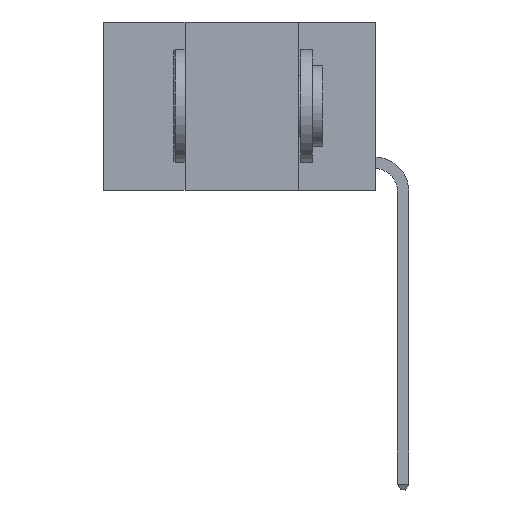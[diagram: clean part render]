
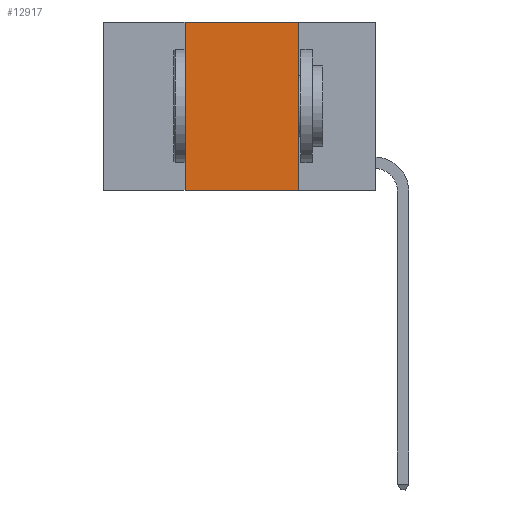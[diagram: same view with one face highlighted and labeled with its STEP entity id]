
A CAD part, left-side view. The second image highlights one B-rep face of the part: STEP entity #12917.
In plain terms, the highlighted planar face has unit normal (-1, 0, 0).
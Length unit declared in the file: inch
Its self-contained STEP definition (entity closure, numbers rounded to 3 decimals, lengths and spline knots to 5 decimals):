
#216 = VERTEX_POINT ( 'NONE', #19023 ) ;
#388 = VERTEX_POINT ( 'NONE', #12282 ) ;
#414 = VERTEX_POINT ( 'NONE', #26466 ) ;
#484 = FACE_OUTER_BOUND ( 'NONE', #21060, .T. ) ;
#968 = CARTESIAN_POINT ( 'NONE',  ( 0., 0.17, 0. ) ) ;
#3764 = VECTOR ( 'NONE', #4431, 39.37008 ) ;
#3788 = EDGE_CURVE ( 'NONE', #414, #388, #21573, .T. ) ;
#4431 = DIRECTION ( 'NONE',  ( 0., -1., 0. ) ) ;
#4776 = DIRECTION ( 'NONE',  ( 0., 0., 1. ) ) ;
#5493 = DIRECTION ( 'NONE',  ( 0., -1., 0. ) ) ;
#6186 = CARTESIAN_POINT ( 'NONE',  ( 0., 0.42, -0.37 ) ) ;
#6542 = VECTOR ( 'NONE', #5493, 39.37008 ) ;
#7232 = LINE ( 'NONE', #15957, #6542 ) ;
#7573 = CARTESIAN_POINT ( 'NONE',  ( 0., 0.6, 0. ) ) ;
#8223 = AXIS2_PLACEMENT_3D ( 'NONE', #7573, #9686, #24364 ) ;
#8956 = CARTESIAN_POINT ( 'NONE',  ( 0., 0.42, 0. ) ) ;
#9109 = ORIENTED_EDGE ( 'NONE', *, *, #15271, .F. ) ;
#9686 = DIRECTION ( 'NONE',  ( 1., 0., 0. ) ) ;
#9690 = DIRECTION ( 'NONE',  ( 0., 0., -1. ) ) ;
#10200 = EDGE_CURVE ( 'NONE', #216, #414, #21294, .T. ) ;
#10779 = VERTEX_POINT ( 'NONE', #6186 ) ;
#12282 = CARTESIAN_POINT ( 'NONE',  ( 0., 0.17, -0.37 ) ) ;
#12917 = ADVANCED_FACE ( 'NONE', ( #484 ), #20148, .F. ) ;
#14665 = ORIENTED_EDGE ( 'NONE', *, *, #3788, .F. ) ;
#15271 = EDGE_CURVE ( 'NONE', #10779, #216, #18026, .T. ) ;
#15783 = ORIENTED_EDGE ( 'NONE', *, *, #26638, .T. ) ;
#15957 = CARTESIAN_POINT ( 'NONE',  ( 0., 0.6, -0.37 ) ) ;
#16601 = VECTOR ( 'NONE', #9690, 39.37008 ) ;
#18026 = LINE ( 'NONE', #8956, #22970 ) ;
#19023 = CARTESIAN_POINT ( 'NONE',  ( 0., 0.42, 0. ) ) ;
#20148 = PLANE ( 'NONE',  #8223 ) ;
#21060 = EDGE_LOOP ( 'NONE', ( #14665, #25829, #9109, #15783 ) ) ;
#21294 = LINE ( 'NONE', #27354, #3764 ) ;
#21573 = LINE ( 'NONE', #968, #16601 ) ;
#22970 = VECTOR ( 'NONE', #4776, 39.37008 ) ;
#24364 = DIRECTION ( 'NONE',  ( 0., 0., -1. ) ) ;
#25829 = ORIENTED_EDGE ( 'NONE', *, *, #10200, .F. ) ;
#26466 = CARTESIAN_POINT ( 'NONE',  ( 0., 0.17, 0. ) ) ;
#26638 = EDGE_CURVE ( 'NONE', #10779, #388, #7232, .T. ) ;
#27354 = CARTESIAN_POINT ( 'NONE',  ( 0., 0.6, 0. ) ) ;
